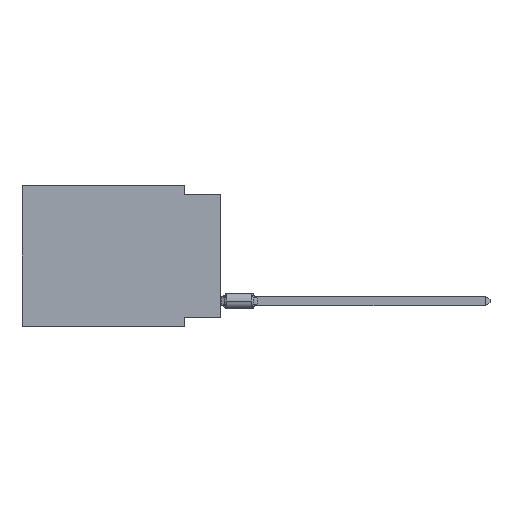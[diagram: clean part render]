
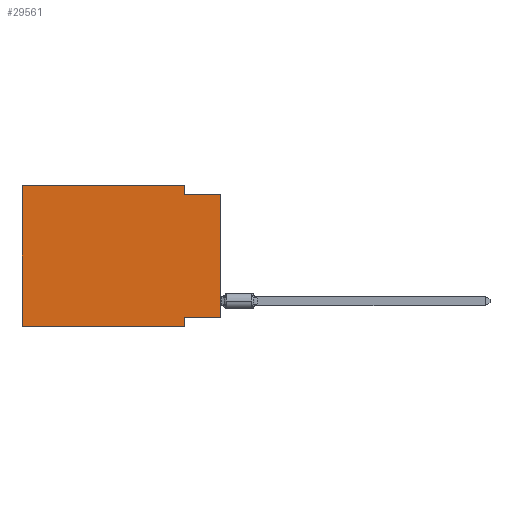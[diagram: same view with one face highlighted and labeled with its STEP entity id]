
A CAD part, left-side view. The second image highlights one B-rep face of the part: STEP entity #29561.
In plain terms, the highlighted planar face has unit normal (-1, 0, 0).
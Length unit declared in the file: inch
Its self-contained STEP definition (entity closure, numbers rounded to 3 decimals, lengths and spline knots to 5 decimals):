
#252 = VECTOR ( 'NONE', #27030, 39.37008 ) ;
#667 = ORIENTED_EDGE ( 'NONE', *, *, #58172, .F. ) ;
#2103 = DIRECTION ( 'NONE',  ( 0., 0., -1. ) ) ;
#5488 = VERTEX_POINT ( 'NONE', #72085 ) ;
#5730 = VERTEX_POINT ( 'NONE', #27963 ) ;
#7124 = LINE ( 'NONE', #48134, #40315 ) ;
#7880 = PLANE ( 'NONE',  #53182 ) ;
#8787 = VECTOR ( 'NONE', #50589, 39.37008 ) ;
#9238 = EDGE_CURVE ( 'NONE', #44937, #5730, #35854, .T. ) ;
#9758 = CARTESIAN_POINT ( 'NONE',  ( 0., 0., -0.365 ) ) ;
#12098 = DIRECTION ( 'NONE',  ( 0., 0., 1. ) ) ;
#12329 = VECTOR ( 'NONE', #73859, 39.37008 ) ;
#13624 = VERTEX_POINT ( 'NONE', #51141 ) ;
#16553 = VECTOR ( 'NONE', #40752, 39.37008 ) ;
#17394 = CARTESIAN_POINT ( 'NONE',  ( 0., 0.1, -0.39 ) ) ;
#19020 = DIRECTION ( 'NONE',  ( 0., 0., -1. ) ) ;
#21661 = CARTESIAN_POINT ( 'NONE',  ( 0., 0., -0.365 ) ) ;
#21762 = CARTESIAN_POINT ( 'NONE',  ( 0., 0.1, -0.39 ) ) ;
#23240 = EDGE_CURVE ( 'NONE', #44937, #48346, #41723, .T. ) ;
#24656 = LINE ( 'NONE', #17394, #16553 ) ;
#24969 = LINE ( 'NONE', #66704, #8787 ) ;
#25450 = VERTEX_POINT ( 'NONE', #26548 ) ;
#26548 = CARTESIAN_POINT ( 'NONE',  ( 0., 0., -0.025 ) ) ;
#27030 = DIRECTION ( 'NONE',  ( 0., -1., 0. ) ) ;
#27963 = CARTESIAN_POINT ( 'NONE',  ( 0., 0.55, 0. ) ) ;
#29561 = ADVANCED_FACE ( 'NONE', ( #48850 ), #7880, .F. ) ;
#30533 = ORIENTED_EDGE ( 'NONE', *, *, #57816, .T. ) ;
#31173 = VECTOR ( 'NONE', #44575, 39.37008 ) ;
#31622 = CARTESIAN_POINT ( 'NONE',  ( 0., 0.55, 0. ) ) ;
#32942 = VERTEX_POINT ( 'NONE', #58181 ) ;
#33891 = VERTEX_POINT ( 'NONE', #9758 ) ;
#35758 = VECTOR ( 'NONE', #12098, 39.37008 ) ;
#35854 = LINE ( 'NONE', #71851, #35758 ) ;
#36163 = CARTESIAN_POINT ( 'NONE',  ( 0., 0.55, -0.39 ) ) ;
#39944 = CARTESIAN_POINT ( 'NONE',  ( 0., 0., 0. ) ) ;
#40315 = VECTOR ( 'NONE', #19020, 39.37008 ) ;
#40752 = DIRECTION ( 'NONE',  ( 0., 0., -1. ) ) ;
#40953 = CARTESIAN_POINT ( 'NONE',  ( 0., 0.55, -0.39 ) ) ;
#41723 = LINE ( 'NONE', #40953, #12329 ) ;
#43897 = LINE ( 'NONE', #67269, #252 ) ;
#44575 = DIRECTION ( 'NONE',  ( 0., 0., 1. ) ) ;
#44937 = VERTEX_POINT ( 'NONE', #36163 ) ;
#45666 = ORIENTED_EDGE ( 'NONE', *, *, #47550, .F. ) ;
#47550 = EDGE_CURVE ( 'NONE', #13624, #25450, #43897, .T. ) ;
#48134 = CARTESIAN_POINT ( 'NONE',  ( 0., 0.1, 0. ) ) ;
#48346 = VERTEX_POINT ( 'NONE', #21762 ) ;
#48565 = ORIENTED_EDGE ( 'NONE', *, *, #23240, .T. ) ;
#48850 = FACE_OUTER_BOUND ( 'NONE', #60150, .T. ) ;
#50589 = DIRECTION ( 'NONE',  ( 0., -1., 0. ) ) ;
#51130 = DIRECTION ( 'NONE',  ( 0., 1., 0. ) ) ;
#51141 = CARTESIAN_POINT ( 'NONE',  ( 0., 0.1, -0.025 ) ) ;
#51750 = EDGE_CURVE ( 'NONE', #33891, #32942, #56914, .T. ) ;
#51867 = VECTOR ( 'NONE', #51130, 39.37008 ) ;
#52524 = EDGE_CURVE ( 'NONE', #5730, #5488, #24969, .T. ) ;
#53182 = AXIS2_PLACEMENT_3D ( 'NONE', #31622, #72239, #2103 ) ;
#54783 = ORIENTED_EDGE ( 'NONE', *, *, #9238, .F. ) ;
#56442 = LINE ( 'NONE', #39944, #31173 ) ;
#56914 = LINE ( 'NONE', #21661, #51867 ) ;
#57816 = EDGE_CURVE ( 'NONE', #33891, #25450, #56442, .T. ) ;
#58172 = EDGE_CURVE ( 'NONE', #32942, #48346, #24656, .T. ) ;
#58181 = CARTESIAN_POINT ( 'NONE',  ( 0., 0.1, -0.365 ) ) ;
#58367 = ORIENTED_EDGE ( 'NONE', *, *, #52524, .F. ) ;
#60150 = EDGE_LOOP ( 'NONE', ( #30533, #45666, #71184, #58367, #54783, #48565, #667, #65043 ) ) ;
#65043 = ORIENTED_EDGE ( 'NONE', *, *, #51750, .F. ) ;
#66704 = CARTESIAN_POINT ( 'NONE',  ( 0., 0.55, 0. ) ) ;
#67269 = CARTESIAN_POINT ( 'NONE',  ( 0., 0., -0.025 ) ) ;
#71184 = ORIENTED_EDGE ( 'NONE', *, *, #72274, .F. ) ;
#71851 = CARTESIAN_POINT ( 'NONE',  ( 0., 0.55, 0. ) ) ;
#72085 = CARTESIAN_POINT ( 'NONE',  ( 0., 0.1, 0. ) ) ;
#72239 = DIRECTION ( 'NONE',  ( 1., 0., 0. ) ) ;
#72274 = EDGE_CURVE ( 'NONE', #5488, #13624, #7124, .T. ) ;
#73859 = DIRECTION ( 'NONE',  ( 0., -1., 0. ) ) ;
